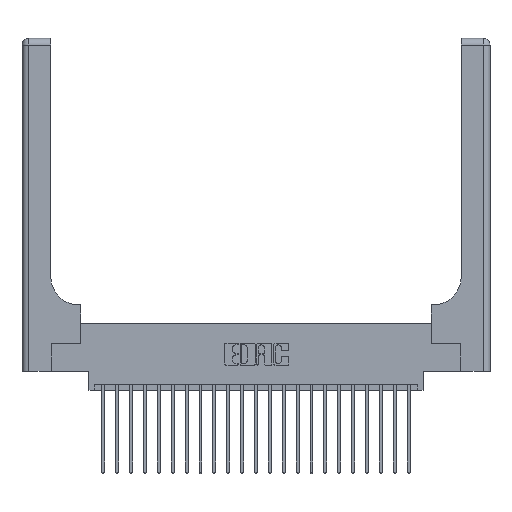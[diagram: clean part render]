
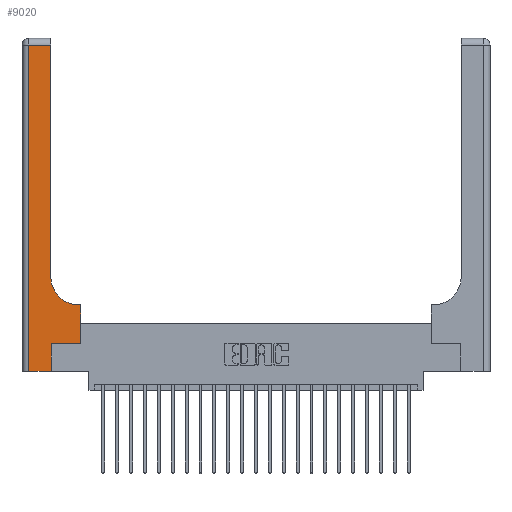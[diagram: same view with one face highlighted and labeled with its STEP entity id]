
A CAD part, top view. The second image highlights one B-rep face of the part: STEP entity #9020.
In plain terms, the highlighted planar face has unit normal (0, 0, 1).
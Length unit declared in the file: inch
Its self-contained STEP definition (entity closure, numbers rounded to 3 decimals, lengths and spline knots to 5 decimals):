
#964 = DIRECTION ( 'NONE',  ( 0., 0., -1. ) ) ;
#1105 = AXIS2_PLACEMENT_3D ( 'NONE', #7241, #3732, #16187 ) ;
#1489 = AXIS2_PLACEMENT_3D ( 'NONE', #11617, #964, #13406 ) ;
#1743 = EDGE_CURVE ( 'NONE', #2025, #21120, #4421, .T. ) ;
#1969 = EDGE_CURVE ( 'NONE', #2146, #2811, #13593, .T. ) ;
#2025 = VERTEX_POINT ( 'NONE', #6538 ) ;
#2109 = EDGE_CURVE ( 'NONE', #2811, #20215, #2462, .T. ) ;
#2114 = VECTOR ( 'NONE', #16220, 39.37008 ) ;
#2146 = VERTEX_POINT ( 'NONE', #5122 ) ;
#2227 = ORIENTED_EDGE ( 'NONE', *, *, #3858, .T. ) ;
#2462 = LINE ( 'NONE', #6765, #11371 ) ;
#2562 = DIRECTION ( 'NONE',  ( -1., 0., 0. ) ) ;
#2583 = EDGE_CURVE ( 'NONE', #12756, #2025, #2991, .T. ) ;
#2778 = ORIENTED_EDGE ( 'NONE', *, *, #1969, .T. ) ;
#2811 = VERTEX_POINT ( 'NONE', #20346 ) ;
#2874 = CARTESIAN_POINT ( 'NONE',  ( 0., 0., 0.37 ) ) ;
#2991 = LINE ( 'NONE', #3819, #11894 ) ;
#3732 = DIRECTION ( 'NONE',  ( 0., 0., -1. ) ) ;
#3819 = CARTESIAN_POINT ( 'NONE',  ( 0.528, 0.25, 0.37 ) ) ;
#3858 = EDGE_CURVE ( 'NONE', #10428, #2146, #11582, .T. ) ;
#4032 = EDGE_LOOP ( 'NONE', ( #15291, #20534, #2227, #2778, #12240, #21638, #12791, #22171, #4452 ) ) ;
#4421 = LINE ( 'NONE', #5536, #22686 ) ;
#4452 = ORIENTED_EDGE ( 'NONE', *, *, #14841, .T. ) ;
#5122 = CARTESIAN_POINT ( 'NONE',  ( 0.06, 0., 0.37 ) ) ;
#5536 = CARTESIAN_POINT ( 'NONE',  ( 0.26, 0.6, 0.37 ) ) ;
#5796 = CARTESIAN_POINT ( 'NONE',  ( 0.265, 0.25, 0.37 ) ) ;
#6538 = CARTESIAN_POINT ( 'NONE',  ( 0.528, 0.6, 0.37 ) ) ;
#6765 = CARTESIAN_POINT ( 'NONE',  ( 0.265, 0., 0.37 ) ) ;
#7241 = CARTESIAN_POINT ( 'NONE',  ( 0., 3., 0.37 ) ) ;
#7587 = DIRECTION ( 'NONE',  ( 1., 0., 0. ) ) ;
#7589 = CARTESIAN_POINT ( 'NONE',  ( 0.06, 2.94, 0.37 ) ) ;
#8013 = EDGE_CURVE ( 'NONE', #20215, #12756, #17805, .T. ) ;
#8097 = FACE_OUTER_BOUND ( 'NONE', #4032, .T. ) ;
#9020 = ADVANCED_FACE ( 'NONE', ( #8097 ), #14389, .F. ) ;
#9153 = CARTESIAN_POINT ( 'NONE',  ( 0.06, 3., 0.37 ) ) ;
#9419 = LINE ( 'NONE', #9633, #18290 ) ;
#9633 = CARTESIAN_POINT ( 'NONE',  ( 0., 2.94, 0.37 ) ) ;
#9782 = DIRECTION ( 'NONE',  ( 0., 1., 0. ) ) ;
#9978 = VECTOR ( 'NONE', #15306, 39.37008 ) ;
#10333 = DIRECTION ( 'NONE',  ( 0., 1., 0. ) ) ;
#10428 = VERTEX_POINT ( 'NONE', #7589 ) ;
#11371 = VECTOR ( 'NONE', #10333, 39.37008 ) ;
#11582 = LINE ( 'NONE', #9153, #2114 ) ;
#11617 = CARTESIAN_POINT ( 'NONE',  ( 0.51, 0.85, 0.37 ) ) ;
#11894 = VECTOR ( 'NONE', #14480, 39.37008 ) ;
#12138 = CIRCLE ( 'NONE', #1489, 0.25 ) ;
#12240 = ORIENTED_EDGE ( 'NONE', *, *, #2109, .T. ) ;
#12425 = CARTESIAN_POINT ( 'NONE',  ( 0.528, 0.25, 0.37 ) ) ;
#12756 = VERTEX_POINT ( 'NONE', #12425 ) ;
#12791 = ORIENTED_EDGE ( 'NONE', *, *, #2583, .T. ) ;
#13021 = LINE ( 'NONE', #18630, #21851 ) ;
#13406 = DIRECTION ( 'NONE',  ( 1., 0., 0. ) ) ;
#13593 = LINE ( 'NONE', #2874, #9978 ) ;
#13813 = CARTESIAN_POINT ( 'NONE',  ( 0.26, 2.94, 0.37 ) ) ;
#14389 = PLANE ( 'NONE',  #1105 ) ;
#14480 = DIRECTION ( 'NONE',  ( 0., 1., 0. ) ) ;
#14841 = EDGE_CURVE ( 'NONE', #21120, #20769, #12138, .T. ) ;
#14970 = CARTESIAN_POINT ( 'NONE',  ( 0.26, 0.85, 0.37 ) ) ;
#15291 = ORIENTED_EDGE ( 'NONE', *, *, #22605, .T. ) ;
#15306 = DIRECTION ( 'NONE',  ( 1., 0., 0. ) ) ;
#16179 = DIRECTION ( 'NONE',  ( -1., 0., 0. ) ) ;
#16182 = VERTEX_POINT ( 'NONE', #13813 ) ;
#16187 = DIRECTION ( 'NONE',  ( -1., 0., 0. ) ) ;
#16220 = DIRECTION ( 'NONE',  ( 0., -1., 0. ) ) ;
#17015 = CARTESIAN_POINT ( 'NONE',  ( 0.265, 0.25, 0.37 ) ) ;
#17260 = VECTOR ( 'NONE', #7587, 39.37008 ) ;
#17805 = LINE ( 'NONE', #5796, #17260 ) ;
#18290 = VECTOR ( 'NONE', #2562, 39.37008 ) ;
#18630 = CARTESIAN_POINT ( 'NONE',  ( 0.26, 3., 0.37 ) ) ;
#20215 = VERTEX_POINT ( 'NONE', #17015 ) ;
#20346 = CARTESIAN_POINT ( 'NONE',  ( 0.265, 0., 0.37 ) ) ;
#20534 = ORIENTED_EDGE ( 'NONE', *, *, #22541, .T. ) ;
#20769 = VERTEX_POINT ( 'NONE', #14970 ) ;
#21120 = VERTEX_POINT ( 'NONE', #21269 ) ;
#21269 = CARTESIAN_POINT ( 'NONE',  ( 0.51, 0.6, 0.37 ) ) ;
#21638 = ORIENTED_EDGE ( 'NONE', *, *, #8013, .T. ) ;
#21851 = VECTOR ( 'NONE', #9782, 39.37008 ) ;
#22171 = ORIENTED_EDGE ( 'NONE', *, *, #1743, .T. ) ;
#22541 = EDGE_CURVE ( 'NONE', #16182, #10428, #9419, .T. ) ;
#22605 = EDGE_CURVE ( 'NONE', #20769, #16182, #13021, .T. ) ;
#22686 = VECTOR ( 'NONE', #16179, 39.37008 ) ;
